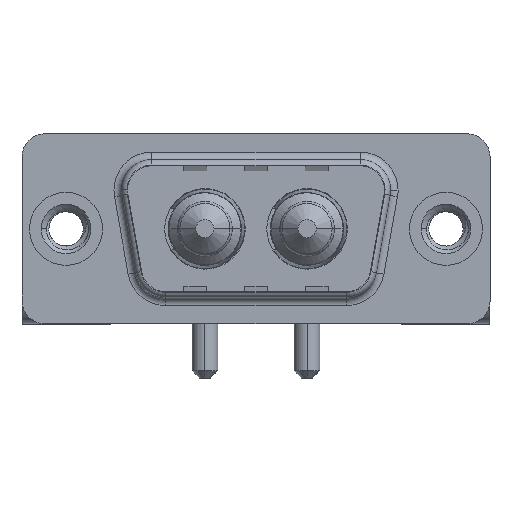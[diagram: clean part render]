
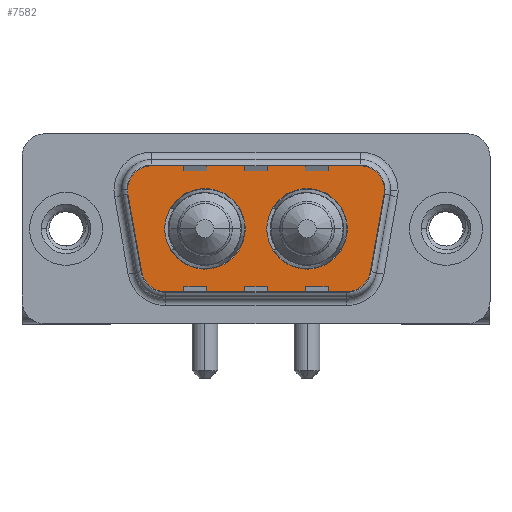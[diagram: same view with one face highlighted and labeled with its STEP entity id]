
A CAD part, top view. The second image highlights one B-rep face of the part: STEP entity #7582.
In plain terms, the highlighted planar face has unit normal (0, 0, 1).
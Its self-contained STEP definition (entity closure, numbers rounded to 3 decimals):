
#81 = CARTESIAN_POINT ( 'NONE',  ( 19.564, 4.9, 0. ) ) ;
#265 = ORIENTED_EDGE ( 'NONE', *, *, #4280, .F. ) ;
#627 = CARTESIAN_POINT ( 'NONE',  ( 18.541, -2.9, 0. ) ) ;
#703 = ORIENTED_EDGE ( 'NONE', *, *, #1387, .T. ) ;
#881 = DIRECTION ( 'NONE',  ( 1., 0., 0. ) ) ;
#994 = VERTEX_POINT ( 'NONE', #10678 ) ;
#1045 = DIRECTION ( 'NONE',  ( 1., 0., 0. ) ) ;
#1169 = VECTOR ( 'NONE', #881, 1000. ) ;
#1265 = VERTEX_POINT ( 'NONE', #6888 ) ;
#1321 = DIRECTION ( 'NONE',  ( 0., 0., 1. ) ) ;
#1366 = CIRCLE ( 'NONE', #8340, 2.65 ) ;
#1387 = EDGE_CURVE ( 'NONE', #1509, #10524, #8503, .T. ) ;
#1459 = AXIS2_PLACEMENT_3D ( 'NONE', #9858, #7821, #8751 ) ;
#1498 = ORIENTED_EDGE ( 'NONE', *, *, #7999, .T. ) ;
#1509 = VERTEX_POINT ( 'NONE', #7930 ) ;
#1523 = ORIENTED_EDGE ( 'NONE', *, *, #6657, .T. ) ;
#1541 = EDGE_CURVE ( 'NONE', #6090, #11437, #12212, .T. ) ;
#1616 = DIRECTION ( 'NONE',  ( 0., 0., 1. ) ) ;
#1638 = EDGE_CURVE ( 'NONE', #8209, #6090, #6235, .T. ) ;
#1766 = CARTESIAN_POINT ( 'NONE',  ( 19.564, 2.9, 0. ) ) ;
#1854 = CARTESIAN_POINT ( 'NONE',  ( 5.436, 4.9, 0. ) ) ;
#1861 = ORIENTED_EDGE ( 'NONE', *, *, #7814, .T. ) ;
#1865 = CARTESIAN_POINT ( 'NONE',  ( 6.49, 0., 0. ) ) ;
#1871 = CARTESIAN_POINT ( 'NONE',  ( 6.459, -4.9, 0. ) ) ;
#1936 = ORIENTED_EDGE ( 'NONE', *, *, #5609, .F. ) ;
#1957 = CARTESIAN_POINT ( 'NONE',  ( 21.534, 2.553, 0. ) ) ;
#1985 = AXIS2_PLACEMENT_3D ( 'NONE', #5644, #12327, #12189 ) ;
#2117 = EDGE_LOOP ( 'NONE', ( #265, #6857 ) ) ;
#2166 = VERTEX_POINT ( 'NONE', #7171 ) ;
#2366 = DIRECTION ( 'NONE',  ( 1., 0., 0. ) ) ;
#3061 = CARTESIAN_POINT ( 'NONE',  ( 4.489, -3.247, 0. ) ) ;
#3228 = EDGE_CURVE ( 'NONE', #6275, #1265, #1366, .T. ) ;
#3340 = AXIS2_PLACEMENT_3D ( 'NONE', #11559, #10567, #2366 ) ;
#3343 = EDGE_LOOP ( 'NONE', ( #1861, #703, #7329, #5581, #6301, #1523, #6993, #8392, #1498 ) ) ;
#3553 = AXIS2_PLACEMENT_3D ( 'NONE', #627, #1616, #4420 ) ;
#3595 = EDGE_CURVE ( 'NONE', #4661, #11164, #4559, .T. ) ;
#4014 = CARTESIAN_POINT ( 'NONE',  ( 15.86, 0., 0. ) ) ;
#4020 = CARTESIAN_POINT ( 'NONE',  ( 9.14, 0., 0. ) ) ;
#4131 = EDGE_CURVE ( 'NONE', #10524, #4661, #7577, .T. ) ;
#4243 = CARTESIAN_POINT ( 'NONE',  ( 21.534, 2.553, 0. ) ) ;
#4280 = EDGE_CURVE ( 'NONE', #6972, #9775, #6777, .T. ) ;
#4420 = DIRECTION ( 'NONE',  ( 1., 0., 0. ) ) ;
#4559 = CIRCLE ( 'NONE', #1985, 2. ) ;
#4661 = VERTEX_POINT ( 'NONE', #9610 ) ;
#4708 = CIRCLE ( 'NONE', #6479, 2.65 ) ;
#5090 = VECTOR ( 'NONE', #6107, 1000. ) ;
#5275 = CARTESIAN_POINT ( 'NONE',  ( 5.436, 2.9, 0. ) ) ;
#5490 = DIRECTION ( 'NONE',  ( 1., 0., 0. ) ) ;
#5504 = PLANE ( 'NONE',  #3340 ) ;
#5581 = ORIENTED_EDGE ( 'NONE', *, *, #3595, .T. ) ;
#5609 = EDGE_CURVE ( 'NONE', #1265, #6275, #4708, .T. ) ;
#5644 = CARTESIAN_POINT ( 'NONE',  ( 19.564, 2.9, 0. ) ) ;
#5784 = AXIS2_PLACEMENT_3D ( 'NONE', #9674, #11372, #8625 ) ;
#6000 = DIRECTION ( 'NONE',  ( 1., 0., 0. ) ) ;
#6090 = VERTEX_POINT ( 'NONE', #3061 ) ;
#6107 = DIRECTION ( 'NONE',  ( 0.174, -0.985, 0. ) ) ;
#6148 = DIRECTION ( 'NONE',  ( 0., 0., 1. ) ) ;
#6217 = CARTESIAN_POINT ( 'NONE',  ( 3.466, 2.553, 0. ) ) ;
#6235 = LINE ( 'NONE', #12023, #5090 ) ;
#6275 = VERTEX_POINT ( 'NONE', #1865 ) ;
#6301 = ORIENTED_EDGE ( 'NONE', *, *, #8427, .T. ) ;
#6414 = ORIENTED_EDGE ( 'NONE', *, *, #3228, .F. ) ;
#6435 = FACE_OUTER_BOUND ( 'NONE', #3343, .T. ) ;
#6479 = AXIS2_PLACEMENT_3D ( 'NONE', #4020, #9581, #1045 ) ;
#6535 = CIRCLE ( 'NONE', #8933, 2.65 ) ;
#6657 = EDGE_CURVE ( 'NONE', #2166, #8209, #7100, .T. ) ;
#6777 = CIRCLE ( 'NONE', #5784, 2.65 ) ;
#6857 = ORIENTED_EDGE ( 'NONE', *, *, #10468, .F. ) ;
#6888 = CARTESIAN_POINT ( 'NONE',  ( 11.79, 0., 0. ) ) ;
#6972 = VERTEX_POINT ( 'NONE', #8643 ) ;
#6993 = ORIENTED_EDGE ( 'NONE', *, *, #1638, .T. ) ;
#7100 = CIRCLE ( 'NONE', #11870, 2. ) ;
#7171 = CARTESIAN_POINT ( 'NONE',  ( 5.436, 4.9, 0. ) ) ;
#7329 = ORIENTED_EDGE ( 'NONE', *, *, #4131, .T. ) ;
#7365 = CARTESIAN_POINT ( 'NONE',  ( 6.459, -4.9, 0. ) ) ;
#7390 = FACE_BOUND ( 'NONE', #2117, .T. ) ;
#7577 = CIRCLE ( 'NONE', #9362, 2. ) ;
#7582 = ADVANCED_FACE ( 'NONE', ( #7390, #11187, #6435 ), #5504, .T. ) ;
#7717 = LINE ( 'NONE', #1854, #8328 ) ;
#7814 = EDGE_CURVE ( 'NONE', #994, #1509, #8743, .T. ) ;
#7821 = DIRECTION ( 'NONE',  ( 0., 0., 1. ) ) ;
#7930 = CARTESIAN_POINT ( 'NONE',  ( 20.511, -3.247, 0. ) ) ;
#7999 = EDGE_CURVE ( 'NONE', #11437, #994, #11462, .T. ) ;
#8209 = VERTEX_POINT ( 'NONE', #6217 ) ;
#8328 = VECTOR ( 'NONE', #10454, 1000. ) ;
#8340 = AXIS2_PLACEMENT_3D ( 'NONE', #9927, #8372, #5490 ) ;
#8372 = DIRECTION ( 'NONE',  ( 0., 0., 1. ) ) ;
#8392 = ORIENTED_EDGE ( 'NONE', *, *, #1541, .T. ) ;
#8427 = EDGE_CURVE ( 'NONE', #11164, #2166, #7717, .T. ) ;
#8503 = LINE ( 'NONE', #1957, #11771 ) ;
#8625 = DIRECTION ( 'NONE',  ( 1., 0., 0. ) ) ;
#8643 = CARTESIAN_POINT ( 'NONE',  ( 18.51, 0., 0. ) ) ;
#8743 = CIRCLE ( 'NONE', #3553, 2. ) ;
#8751 = DIRECTION ( 'NONE',  ( -1., 0., 0. ) ) ;
#8933 = AXIS2_PLACEMENT_3D ( 'NONE', #4014, #1321, #6000 ) ;
#9244 = DIRECTION ( 'NONE',  ( -1., 0., 0. ) ) ;
#9362 = AXIS2_PLACEMENT_3D ( 'NONE', #1766, #12036, #9244 ) ;
#9581 = DIRECTION ( 'NONE',  ( 0., 0., 1. ) ) ;
#9610 = CARTESIAN_POINT ( 'NONE',  ( 21.564, 2.9, 0. ) ) ;
#9614 = EDGE_LOOP ( 'NONE', ( #1936, #6414 ) ) ;
#9674 = CARTESIAN_POINT ( 'NONE',  ( 15.86, 0., 0. ) ) ;
#9775 = VERTEX_POINT ( 'NONE', #11333 ) ;
#9858 = CARTESIAN_POINT ( 'NONE',  ( 6.459, -2.9, 0. ) ) ;
#9927 = CARTESIAN_POINT ( 'NONE',  ( 9.14, 0., 0. ) ) ;
#10454 = DIRECTION ( 'NONE',  ( -1., 0., 0. ) ) ;
#10468 = EDGE_CURVE ( 'NONE', #9775, #6972, #6535, .T. ) ;
#10524 = VERTEX_POINT ( 'NONE', #4243 ) ;
#10567 = DIRECTION ( 'NONE',  ( 0., 0., 1. ) ) ;
#10678 = CARTESIAN_POINT ( 'NONE',  ( 18.541, -4.9, 0. ) ) ;
#11164 = VERTEX_POINT ( 'NONE', #81 ) ;
#11187 = FACE_BOUND ( 'NONE', #9614, .T. ) ;
#11333 = CARTESIAN_POINT ( 'NONE',  ( 13.21, 0., 0. ) ) ;
#11372 = DIRECTION ( 'NONE',  ( 0., 0., 1. ) ) ;
#11437 = VERTEX_POINT ( 'NONE', #7365 ) ;
#11462 = LINE ( 'NONE', #1871, #1169 ) ;
#11559 = CARTESIAN_POINT ( 'NONE',  ( 18.541, -2.9, 0. ) ) ;
#11771 = VECTOR ( 'NONE', #12304, 1000. ) ;
#11870 = AXIS2_PLACEMENT_3D ( 'NONE', #5275, #6148, #11872 ) ;
#11872 = DIRECTION ( 'NONE',  ( 1., 0., 0. ) ) ;
#12023 = CARTESIAN_POINT ( 'NONE',  ( 3.466, 2.553, 0. ) ) ;
#12036 = DIRECTION ( 'NONE',  ( 0., 0., 1. ) ) ;
#12189 = DIRECTION ( 'NONE',  ( -1., 0., 0. ) ) ;
#12212 = CIRCLE ( 'NONE', #1459, 2. ) ;
#12304 = DIRECTION ( 'NONE',  ( 0.174, 0.985, 0. ) ) ;
#12327 = DIRECTION ( 'NONE',  ( 0., 0., 1. ) ) ;
